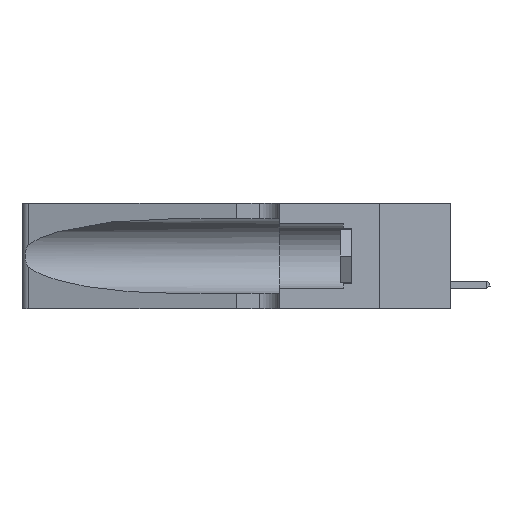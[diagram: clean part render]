
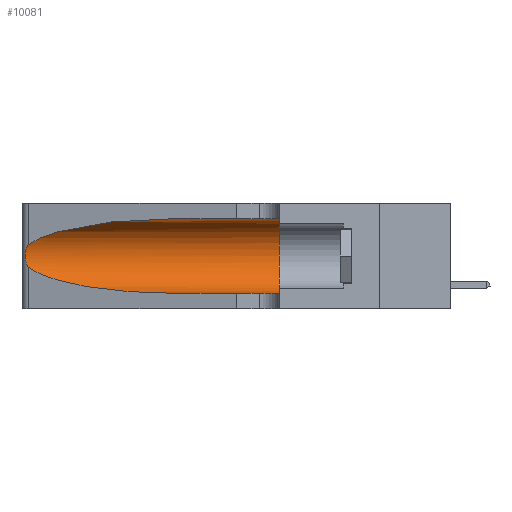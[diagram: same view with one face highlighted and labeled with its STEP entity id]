
A CAD part, left-side view. The second image highlights one B-rep face of the part: STEP entity #10081.
In plain terms, the highlighted cylindrical face has radius 3.308 mm (diameter 6.617 mm), a partial arc.
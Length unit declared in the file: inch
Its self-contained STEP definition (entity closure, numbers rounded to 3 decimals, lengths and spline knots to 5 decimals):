
#1188 = CARTESIAN_POINT ( 'NONE',  ( 0.1305, 0.72297, 0.31525 ) ) ;
#1557 = CARTESIAN_POINT ( 'NONE',  ( 0.26017, 1.23833, 0.17102 ) ) ;
#1858 = EDGE_CURVE ( 'NONE', #26964, #2198, #27487, .T. ) ;
#2198 = VERTEX_POINT ( 'NONE', #22748 ) ;
#3824 = CARTESIAN_POINT ( 'NONE',  ( 0.25854, 1.2359, 0.20912 ) ) ;
#3955 = B_SPLINE_CURVE_WITH_KNOTS ( 'NONE', 3,
 ( #25872, #19091, #4178, #23189, #3824, #10035, #25923, #22989, #1557, #7245, #15117, #14377, #5250, #20746 ),
 .UNSPECIFIED., .F., .F.,
 ( 4, 2, 2, 2, 2, 2, 4 ),
 ( 0., 0.00027, 0.00053, 0.00107, 0.0016, 0.00187, 0.00214 ),
 .UNSPECIFIED. ) ;
#4178 = CARTESIAN_POINT ( 'NONE',  ( 0.25639, 1.23184, 0.21858 ) ) ;
#5250 = CARTESIAN_POINT ( 'NONE',  ( 0.25555, 1.22993, 0.14849 ) ) ;
#5616 = DIRECTION ( 'NONE',  ( 0., -1., 0. ) ) ;
#5691 = DIRECTION ( 'NONE',  ( 0., -1., 0. ) ) ;
#6427 = CARTESIAN_POINT ( 'NONE',  ( 0.1305, 0.72297, 0.31525 ) ) ;
#6437 = LINE ( 'NONE', #14667, #23577 ) ;
#6781 = EDGE_CURVE ( 'NONE', #17575, #2198, #6437, .T. ) ;
#7107 = ORIENTED_EDGE ( 'NONE', *, *, #1858, .F. ) ;
#7113 = ORIENTED_EDGE ( 'NONE', *, *, #15522, .T. ) ;
#7245 = CARTESIAN_POINT ( 'NONE',  ( 0.25856, 1.23593, 0.16098 ) ) ;
#9639 = VERTEX_POINT ( 'NONE', #6427 ) ;
#10035 = CARTESIAN_POINT ( 'NONE',  ( 0.26018, 1.23835, 0.19895 ) ) ;
#10081 = ADVANCED_FACE ( 'NONE', ( #28295 ), #12203, .F. ) ;
#10111 = DIRECTION ( 'NONE',  ( 0., 0., -1. ) ) ;
#10137 = CARTESIAN_POINT ( 'NONE',  ( 0.2373, 1.15595, 0.28018 ) ) ;
#11761 =( BOUNDED_CURVE ( )  B_SPLINE_CURVE ( 3, ( #1188, #18995, #10137, #14414 ),
 .UNSPECIFIED., .F., .F. ) 
 B_SPLINE_CURVE_WITH_KNOTS ( ( 4, 4 ),
 ( 1.5708, 2.84003 ),
 .UNSPECIFIED. ) 
 CURVE ( )  GEOMETRIC_REPRESENTATION_ITEM ( )  RATIONAL_B_SPLINE_CURVE ( ( 1., 0.87, 0.87, 1. ) ) 
 REPRESENTATION_ITEM ( '' )  );
#11850 = CARTESIAN_POINT ( 'NONE',  ( 0.1305, 1.61858, 0.31525 ) ) ;
#12143 = CARTESIAN_POINT ( 'NONE',  ( 0.25487, 1.22718, 0.14631 ) ) ;
#12203 = CYLINDRICAL_SURFACE ( 'NONE', #15394, 0.13025 ) ;
#12452 = EDGE_CURVE ( 'NONE', #27144, #17575, #20020, .T. ) ;
#12609 = CARTESIAN_POINT ( 'NONE',  ( 0.25487, 1.22718, 0.14631 ) ) ;
#12752 = EDGE_LOOP ( 'NONE', ( #7113, #22742, #27285, #21234, #7107, #13781 ) ) ;
#13420 = EDGE_CURVE ( 'NONE', #24313, #27144, #3955, .T. ) ;
#13781 = ORIENTED_EDGE ( 'NONE', *, *, #27989, .F. ) ;
#14377 = CARTESIAN_POINT ( 'NONE',  ( 0.25639, 1.23186, 0.15144 ) ) ;
#14407 = CARTESIAN_POINT ( 'NONE',  ( 0.2373, 1.15595, 0.08982 ) ) ;
#14414 = CARTESIAN_POINT ( 'NONE',  ( 0.25487, 1.22718, 0.22369 ) ) ;
#14667 = CARTESIAN_POINT ( 'NONE',  ( 0.1305, 1.61858, 0.05475 ) ) ;
#15028 = CARTESIAN_POINT ( 'NONE',  ( 0.1305, 0.72297, 0.05475 ) ) ;
#15039 = AXIS2_PLACEMENT_3D ( 'NONE', #28429, #23855, #24237 ) ;
#15117 = CARTESIAN_POINT ( 'NONE',  ( 0.25789, 1.23486, 0.15765 ) ) ;
#15394 = AXIS2_PLACEMENT_3D ( 'NONE', #18869, #5691, #10111 ) ;
#15522 = EDGE_CURVE ( 'NONE', #9639, #24313, #11761, .T. ) ;
#15875 = LINE ( 'NONE', #11850, #25289 ) ;
#16685 = CARTESIAN_POINT ( 'NONE',  ( 0.1305, 0.72297, 0.05475 ) ) ;
#16775 = CARTESIAN_POINT ( 'NONE',  ( 0.18966, 0.96281, 0.05475 ) ) ;
#17575 = VERTEX_POINT ( 'NONE', #15028 ) ;
#18869 = CARTESIAN_POINT ( 'NONE',  ( 0.1305, 1.61858, 0.185 ) ) ;
#18995 = CARTESIAN_POINT ( 'NONE',  ( 0.18966, 0.96281, 0.31525 ) ) ;
#19091 = CARTESIAN_POINT ( 'NONE',  ( 0.25555, 1.22994, 0.2215 ) ) ;
#20020 =( BOUNDED_CURVE ( )  B_SPLINE_CURVE ( 3, ( #12143, #14407, #16775, #16685 ),
 .UNSPECIFIED., .F., .F. ) 
 B_SPLINE_CURVE_WITH_KNOTS ( ( 4, 4 ),
 ( 3.44316, 4.71239 ),
 .UNSPECIFIED. ) 
 CURVE ( )  GEOMETRIC_REPRESENTATION_ITEM ( )  RATIONAL_B_SPLINE_CURVE ( ( 1., 0.87, 0.87, 1. ) ) 
 REPRESENTATION_ITEM ( '' )  );
#20746 = CARTESIAN_POINT ( 'NONE',  ( 0.25487, 1.22718, 0.14631 ) ) ;
#21234 = ORIENTED_EDGE ( 'NONE', *, *, #6781, .T. ) ;
#22554 = CARTESIAN_POINT ( 'NONE',  ( 0.25487, 1.22718, 0.22369 ) ) ;
#22742 = ORIENTED_EDGE ( 'NONE', *, *, #13420, .T. ) ;
#22748 = CARTESIAN_POINT ( 'NONE',  ( 0.1305, 0.35, 0.05475 ) ) ;
#22989 = CARTESIAN_POINT ( 'NONE',  ( 0.26075, 1.23896, 0.178 ) ) ;
#23189 = CARTESIAN_POINT ( 'NONE',  ( 0.25787, 1.23484, 0.2124 ) ) ;
#23577 = VECTOR ( 'NONE', #27851, 39.37008 ) ;
#23855 = DIRECTION ( 'NONE',  ( 0., 1., 0. ) ) ;
#24237 = DIRECTION ( 'NONE',  ( 0., 0., 1. ) ) ;
#24313 = VERTEX_POINT ( 'NONE', #22554 ) ;
#25289 = VECTOR ( 'NONE', #5616, 39.37008 ) ;
#25872 = CARTESIAN_POINT ( 'NONE',  ( 0.25487, 1.22718, 0.22369 ) ) ;
#25923 = CARTESIAN_POINT ( 'NONE',  ( 0.26075, 1.23896, 0.19203 ) ) ;
#26964 = VERTEX_POINT ( 'NONE', #27824 ) ;
#27144 = VERTEX_POINT ( 'NONE', #12609 ) ;
#27285 = ORIENTED_EDGE ( 'NONE', *, *, #12452, .T. ) ;
#27487 = CIRCLE ( 'NONE', #15039, 0.13025 ) ;
#27824 = CARTESIAN_POINT ( 'NONE',  ( 0.1305, 0.35, 0.31525 ) ) ;
#27851 = DIRECTION ( 'NONE',  ( 0., -1., 0. ) ) ;
#27989 = EDGE_CURVE ( 'NONE', #9639, #26964, #15875, .T. ) ;
#28295 = FACE_OUTER_BOUND ( 'NONE', #12752, .T. ) ;
#28429 = CARTESIAN_POINT ( 'NONE',  ( 0.1305, 0.35, 0.185 ) ) ;
